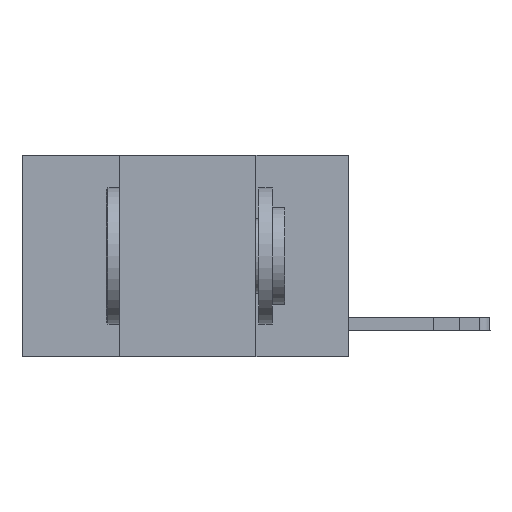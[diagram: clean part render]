
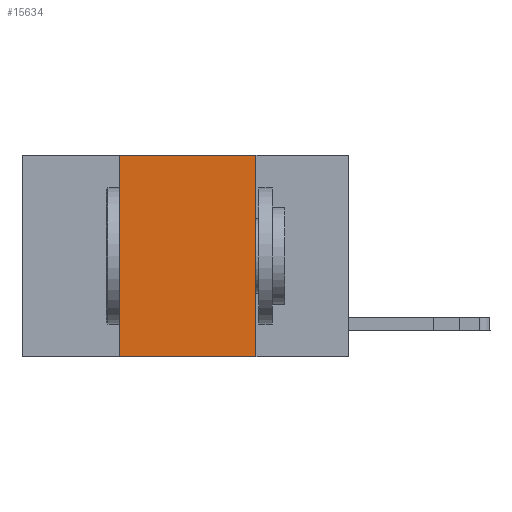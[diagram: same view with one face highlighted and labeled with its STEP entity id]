
A CAD part, left-side view. The second image highlights one B-rep face of the part: STEP entity #15634.
In plain terms, the highlighted planar face has unit normal (-1, 0, 0).
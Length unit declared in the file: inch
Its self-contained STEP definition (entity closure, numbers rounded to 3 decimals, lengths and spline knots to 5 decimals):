
#885 = FACE_OUTER_BOUND ( 'NONE', #15953, .T. ) ;
#927 = ORIENTED_EDGE ( 'NONE', *, *, #8274, .F. ) ;
#1672 = AXIS2_PLACEMENT_3D ( 'NONE', #13243, #4763, #10295 ) ;
#2067 = CARTESIAN_POINT ( 'NONE',  ( 0., 0.42, -0.37 ) ) ;
#2090 = VERTEX_POINT ( 'NONE', #14798 ) ;
#2341 = DIRECTION ( 'NONE',  ( 0., 0., 1. ) ) ;
#2474 = VECTOR ( 'NONE', #4351, 39.37008 ) ;
#3266 = VERTEX_POINT ( 'NONE', #8973 ) ;
#4351 = DIRECTION ( 'NONE',  ( 0., -1., 0. ) ) ;
#4763 = DIRECTION ( 'NONE',  ( 1., 0., 0. ) ) ;
#5087 = ORIENTED_EDGE ( 'NONE', *, *, #15709, .F. ) ;
#5198 = EDGE_CURVE ( 'NONE', #5844, #2090, #12638, .T. ) ;
#5844 = VERTEX_POINT ( 'NONE', #2067 ) ;
#6588 = CARTESIAN_POINT ( 'NONE',  ( 0., 0.42, 0. ) ) ;
#7075 = VERTEX_POINT ( 'NONE', #12805 ) ;
#8213 = VECTOR ( 'NONE', #12550, 39.37008 ) ;
#8274 = EDGE_CURVE ( 'NONE', #3266, #7075, #14101, .T. ) ;
#8973 = CARTESIAN_POINT ( 'NONE',  ( 0., 0.42, 0. ) ) ;
#10295 = DIRECTION ( 'NONE',  ( 0., 0., -1. ) ) ;
#10374 = ORIENTED_EDGE ( 'NONE', *, *, #5198, .T. ) ;
#10494 = LINE ( 'NONE', #6588, #17933 ) ;
#10662 = LINE ( 'NONE', #17698, #17927 ) ;
#10923 = DIRECTION ( 'NONE',  ( 0., 0., -1. ) ) ;
#11502 = EDGE_CURVE ( 'NONE', #5844, #3266, #10494, .T. ) ;
#12550 = DIRECTION ( 'NONE',  ( 0., -1., 0. ) ) ;
#12638 = LINE ( 'NONE', #15377, #8213 ) ;
#12805 = CARTESIAN_POINT ( 'NONE',  ( 0., 0.17, 0. ) ) ;
#13243 = CARTESIAN_POINT ( 'NONE',  ( 0., 0.6, 0. ) ) ;
#13333 = PLANE ( 'NONE',  #1672 ) ;
#14101 = LINE ( 'NONE', #16744, #2474 ) ;
#14798 = CARTESIAN_POINT ( 'NONE',  ( 0., 0.17, -0.37 ) ) ;
#15377 = CARTESIAN_POINT ( 'NONE',  ( 0., 0.6, -0.37 ) ) ;
#15634 = ADVANCED_FACE ( 'NONE', ( #885 ), #13333, .F. ) ;
#15709 = EDGE_CURVE ( 'NONE', #7075, #2090, #10662, .T. ) ;
#15953 = EDGE_LOOP ( 'NONE', ( #5087, #927, #16598, #10374 ) ) ;
#16598 = ORIENTED_EDGE ( 'NONE', *, *, #11502, .F. ) ;
#16744 = CARTESIAN_POINT ( 'NONE',  ( 0., 0.6, 0. ) ) ;
#17698 = CARTESIAN_POINT ( 'NONE',  ( 0., 0.17, 0. ) ) ;
#17927 = VECTOR ( 'NONE', #10923, 39.37008 ) ;
#17933 = VECTOR ( 'NONE', #2341, 39.37008 ) ;
